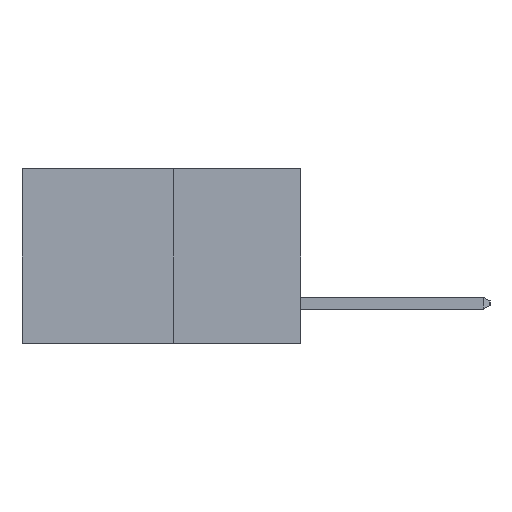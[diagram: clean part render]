
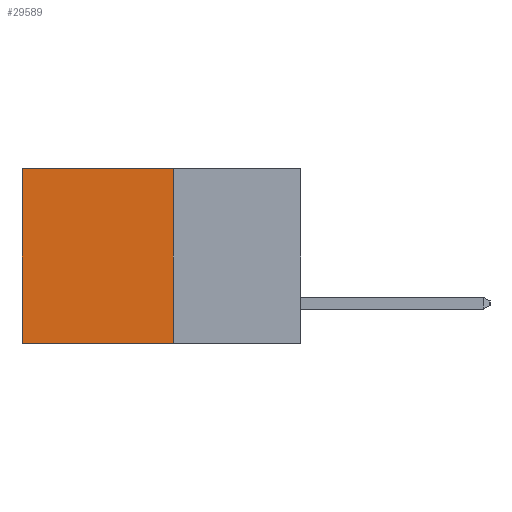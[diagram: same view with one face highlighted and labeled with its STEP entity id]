
A CAD part, left-side view. The second image highlights one B-rep face of the part: STEP entity #29589.
In plain terms, the highlighted planar face has unit normal (-1, 0, 0).
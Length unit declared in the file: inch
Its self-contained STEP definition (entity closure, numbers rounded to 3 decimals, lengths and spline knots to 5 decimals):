
#231 = ORIENTED_EDGE ( 'NONE', *, *, #23911, .F. ) ;
#808 = VECTOR ( 'NONE', #24247, 39.37008 ) ;
#1617 = CARTESIAN_POINT ( 'NONE',  ( 0.277, 0.27, 0. ) ) ;
#2148 = LINE ( 'NONE', #1617, #28745 ) ;
#2656 = PLANE ( 'NONE',  #7922 ) ;
#2768 = DIRECTION ( 'NONE',  ( 0., 0., -1. ) ) ;
#3704 = CARTESIAN_POINT ( 'NONE',  ( 0.277, 0.27, -0.37 ) ) ;
#3924 = LINE ( 'NONE', #7914, #30464 ) ;
#5398 = ORIENTED_EDGE ( 'NONE', *, *, #15265, .T. ) ;
#5970 = EDGE_CURVE ( 'NONE', #10483, #25452, #8675, .T. ) ;
#6162 = EDGE_LOOP ( 'NONE', ( #30327, #231, #26613, #5398 ) ) ;
#7021 = CARTESIAN_POINT ( 'NONE',  ( 0.277, 0.27, 0. ) ) ;
#7914 = CARTESIAN_POINT ( 'NONE',  ( 0.277, 0.27, -0.37 ) ) ;
#7922 = AXIS2_PLACEMENT_3D ( 'NONE', #10500, #18224, #2768 ) ;
#8675 = LINE ( 'NONE', #13400, #22366 ) ;
#10483 = VERTEX_POINT ( 'NONE', #18211 ) ;
#10500 = CARTESIAN_POINT ( 'NONE',  ( 0.277, 0.27, -0.37 ) ) ;
#12066 = VERTEX_POINT ( 'NONE', #15639 ) ;
#13400 = CARTESIAN_POINT ( 'NONE',  ( 0.277, 0.59, -0.37 ) ) ;
#13842 = DIRECTION ( 'NONE',  ( 0., 0., -1. ) ) ;
#15265 = EDGE_CURVE ( 'NONE', #24859, #10483, #2148, .T. ) ;
#15639 = CARTESIAN_POINT ( 'NONE',  ( 0.277, 0.27, -0.37 ) ) ;
#18211 = CARTESIAN_POINT ( 'NONE',  ( 0.277, 0.59, 0. ) ) ;
#18224 = DIRECTION ( 'NONE',  ( 1., 0., 0. ) ) ;
#21597 = EDGE_CURVE ( 'NONE', #24859, #12066, #28178, .T. ) ;
#22366 = VECTOR ( 'NONE', #13842, 39.37008 ) ;
#23329 = DIRECTION ( 'NONE',  ( 0., 1., 0. ) ) ;
#23666 = FACE_OUTER_BOUND ( 'NONE', #6162, .T. ) ;
#23911 = EDGE_CURVE ( 'NONE', #12066, #25452, #3924, .T. ) ;
#24247 = DIRECTION ( 'NONE',  ( 0., 0., -1. ) ) ;
#24856 = DIRECTION ( 'NONE',  ( 0., 1., 0. ) ) ;
#24859 = VERTEX_POINT ( 'NONE', #7021 ) ;
#25313 = CARTESIAN_POINT ( 'NONE',  ( 0.277, 0.59, -0.37 ) ) ;
#25452 = VERTEX_POINT ( 'NONE', #25313 ) ;
#26613 = ORIENTED_EDGE ( 'NONE', *, *, #21597, .F. ) ;
#28178 = LINE ( 'NONE', #3704, #808 ) ;
#28745 = VECTOR ( 'NONE', #24856, 39.37008 ) ;
#29589 = ADVANCED_FACE ( 'NONE', ( #23666 ), #2656, .F. ) ;
#30327 = ORIENTED_EDGE ( 'NONE', *, *, #5970, .T. ) ;
#30464 = VECTOR ( 'NONE', #23329, 39.37008 ) ;
